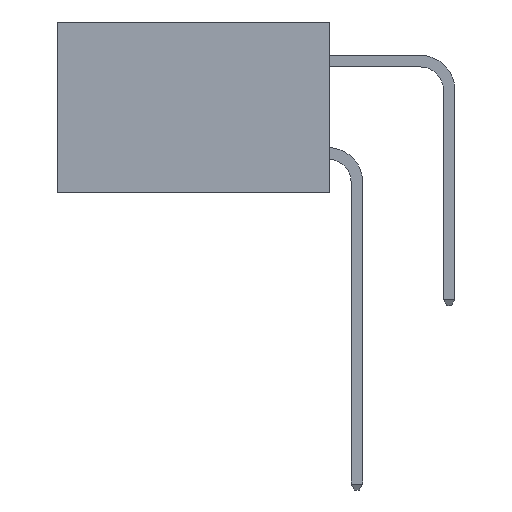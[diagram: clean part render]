
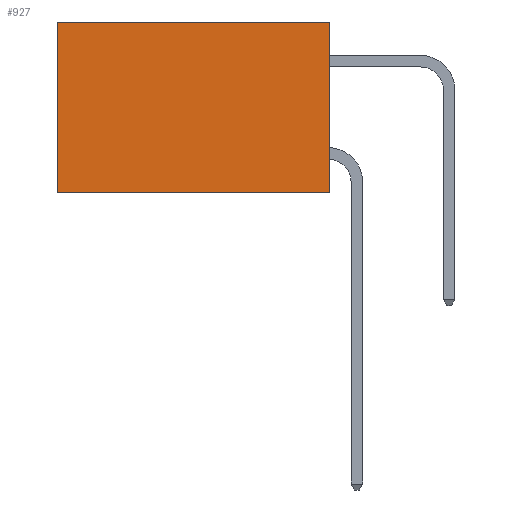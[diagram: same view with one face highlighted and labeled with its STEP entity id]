
A CAD part, left-side view. The second image highlights one B-rep face of the part: STEP entity #927.
In plain terms, the highlighted planar face has unit normal (-1, 0, 0).
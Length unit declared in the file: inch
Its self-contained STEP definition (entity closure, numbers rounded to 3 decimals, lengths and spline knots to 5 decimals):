
#514 = CARTESIAN_POINT ( 'NONE',  ( 0.277, 0., -0.37 ) ) ;
#783 = VERTEX_POINT ( 'NONE', #7482 ) ;
#927 = ADVANCED_FACE ( 'NONE', ( #11594 ), #4456, .F. ) ;
#1065 = EDGE_CURVE ( 'NONE', #3734, #10044, #9063, .T. ) ;
#1107 = CARTESIAN_POINT ( 'NONE',  ( 0.277, 0., 0. ) ) ;
#1531 = LINE ( 'NONE', #3432, #6778 ) ;
#1868 = CARTESIAN_POINT ( 'NONE',  ( 0.277, 0., 0. ) ) ;
#2475 = DIRECTION ( 'NONE',  ( 0., 0., -1. ) ) ;
#2516 = LINE ( 'NONE', #9736, #7732 ) ;
#2928 = AXIS2_PLACEMENT_3D ( 'NONE', #514, #8529, #8269 ) ;
#3190 = CARTESIAN_POINT ( 'NONE',  ( 0.277, 0., -0.37 ) ) ;
#3432 = CARTESIAN_POINT ( 'NONE',  ( 0.277, 0., -0.37 ) ) ;
#3540 = EDGE_CURVE ( 'NONE', #3734, #10073, #12150, .T. ) ;
#3734 = VERTEX_POINT ( 'NONE', #1868 ) ;
#3855 = DIRECTION ( 'NONE',  ( 0., 1., 0. ) ) ;
#3915 = VECTOR ( 'NONE', #5188, 39.37008 ) ;
#4456 = PLANE ( 'NONE',  #2928 ) ;
#4877 = EDGE_LOOP ( 'NONE', ( #6711, #7032, #7153, #7335 ) ) ;
#5188 = DIRECTION ( 'NONE',  ( 0., 0., -1. ) ) ;
#5460 = CARTESIAN_POINT ( 'NONE',  ( 0.277, 0., -0.37 ) ) ;
#6285 = VECTOR ( 'NONE', #3855, 39.37008 ) ;
#6711 = ORIENTED_EDGE ( 'NONE', *, *, #12245, .T. ) ;
#6778 = VECTOR ( 'NONE', #11709, 39.37008 ) ;
#7032 = ORIENTED_EDGE ( 'NONE', *, *, #11204, .F. ) ;
#7153 = ORIENTED_EDGE ( 'NONE', *, *, #3540, .F. ) ;
#7335 = ORIENTED_EDGE ( 'NONE', *, *, #1065, .T. ) ;
#7482 = CARTESIAN_POINT ( 'NONE',  ( 0.277, 0.59, -0.37 ) ) ;
#7732 = VECTOR ( 'NONE', #2475, 39.37008 ) ;
#8269 = DIRECTION ( 'NONE',  ( 0., 0., -1. ) ) ;
#8529 = DIRECTION ( 'NONE',  ( 1., 0., 0. ) ) ;
#9063 = LINE ( 'NONE', #1107, #6285 ) ;
#9736 = CARTESIAN_POINT ( 'NONE',  ( 0.277, 0.59, -0.37 ) ) ;
#10044 = VERTEX_POINT ( 'NONE', #12398 ) ;
#10073 = VERTEX_POINT ( 'NONE', #3190 ) ;
#11204 = EDGE_CURVE ( 'NONE', #10073, #783, #1531, .T. ) ;
#11594 = FACE_OUTER_BOUND ( 'NONE', #4877, .T. ) ;
#11709 = DIRECTION ( 'NONE',  ( 0., 1., 0. ) ) ;
#12150 = LINE ( 'NONE', #5460, #3915 ) ;
#12245 = EDGE_CURVE ( 'NONE', #10044, #783, #2516, .T. ) ;
#12398 = CARTESIAN_POINT ( 'NONE',  ( 0.277, 0.59, 0. ) ) ;
